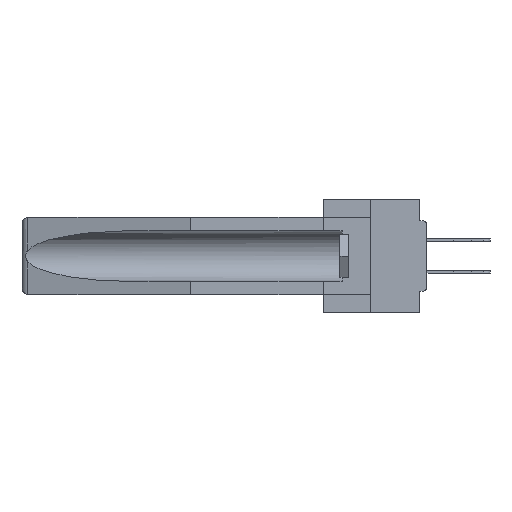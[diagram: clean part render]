
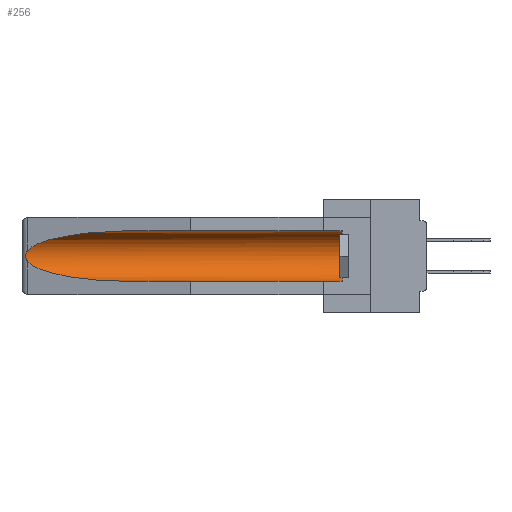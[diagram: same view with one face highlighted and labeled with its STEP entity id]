
A CAD part, left-side view. The second image highlights one B-rep face of the part: STEP entity #256.
In plain terms, the highlighted cylindrical face has radius 2.857 mm (diameter 5.715 mm), a partial arc.
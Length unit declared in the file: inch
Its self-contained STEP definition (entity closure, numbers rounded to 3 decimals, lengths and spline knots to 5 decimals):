
#256 = ADVANCED_FACE ( 'NONE', ( #24454 ), #22703, .F. ) ;
#654 = VERTEX_POINT ( 'NONE', #26336 ) ;
#983 = EDGE_CURVE ( 'NONE', #9670, #654, #21777, .T. ) ;
#1067 = LINE ( 'NONE', #14874, #6768 ) ;
#1359 = CARTESIAN_POINT ( 'NONE',  ( 0.26537, 1.52718, -0.14972 ) ) ;
#2585 = VERTEX_POINT ( 'NONE', #13475 ) ;
#2924 = CARTESIAN_POINT ( 'NONE',  ( 0.155, 0.126, -0.1715 ) ) ;
#4536 = CARTESIAN_POINT ( 'NONE',  ( 0.2675, 1.53308, -0.16763 ) ) ;
#6568 =( BOUNDED_CURVE ( )  B_SPLINE_CURVE ( 3, ( #15482, #18319, #7255, #1359 ),
 .UNSPECIFIED., .F., .F. ) 
 B_SPLINE_CURVE_WITH_KNOTS ( ( 4, 4 ),
 ( 4.71239, 6.08839 ),
 .UNSPECIFIED. ) 
 CURVE ( )  GEOMETRIC_REPRESENTATION_ITEM ( )  RATIONAL_B_SPLINE_CURVE ( ( 1., 0.848, 0.848, 1. ) ) 
 REPRESENTATION_ITEM ( '' )  );
#6768 = VECTOR ( 'NONE', #34058, 39.37008 ) ;
#7037 = DIRECTION ( 'NONE',  ( 0., 1., 0. ) ) ;
#7255 = CARTESIAN_POINT ( 'NONE',  ( 0.25451, 1.48313, -0.09465 ) ) ;
#8725 = CARTESIAN_POINT ( 'NONE',  ( 0.155, 0.126, -0.284 ) ) ;
#9670 = VERTEX_POINT ( 'NONE', #8725 ) ;
#9935 = CARTESIAN_POINT ( 'NONE',  ( 0.2675, 1.53308, -0.17534 ) ) ;
#10050 = CARTESIAN_POINT ( 'NONE',  ( 0.2673, 1.53269, -0.17917 ) ) ;
#10178 = CARTESIAN_POINT ( 'NONE',  ( 0.26654, 1.53092, -0.15636 ) ) ;
#10819 = EDGE_CURVE ( 'NONE', #2585, #19318, #11985, .T. ) ;
#11294 = DIRECTION ( 'NONE',  ( 0., -1., 0. ) ) ;
#11563 = ORIENTED_EDGE ( 'NONE', *, *, #10819, .T. ) ;
#11985 =( BOUNDED_CURVE ( )  B_SPLINE_CURVE ( 3, ( #14774, #20564, #17224, #28780 ),
 .UNSPECIFIED., .F., .F. ) 
 B_SPLINE_CURVE_WITH_KNOTS ( ( 4, 4 ),
 ( 0.1948, 1.5708 ),
 .UNSPECIFIED. ) 
 CURVE ( )  GEOMETRIC_REPRESENTATION_ITEM ( )  RATIONAL_B_SPLINE_CURVE ( ( 1., 0.848, 0.848, 1. ) ) 
 REPRESENTATION_ITEM ( '' )  );
#12118 = VERTEX_POINT ( 'NONE', #25406 ) ;
#12431 = AXIS2_PLACEMENT_3D ( 'NONE', #2924, #11294, #33782 ) ;
#12570 = CARTESIAN_POINT ( 'NONE',  ( 0.155, -0.30754, -0.059 ) ) ;
#13475 = CARTESIAN_POINT ( 'NONE',  ( 0.26537, 1.52718, -0.19328 ) ) ;
#14332 = AXIS2_PLACEMENT_3D ( 'NONE', #29173, #26584, #31389 ) ;
#14689 = ORIENTED_EDGE ( 'NONE', *, *, #23498, .T. ) ;
#14774 = CARTESIAN_POINT ( 'NONE',  ( 0.26537, 1.52718, -0.19328 ) ) ;
#14874 = CARTESIAN_POINT ( 'NONE',  ( 0.155, -0.30754, -0.284 ) ) ;
#15314 = ORIENTED_EDGE ( 'NONE', *, *, #983, .T. ) ;
#15482 = CARTESIAN_POINT ( 'NONE',  ( 0.155, 1.07973, -0.059 ) ) ;
#15732 = CARTESIAN_POINT ( 'NONE',  ( 0.26655, 1.53094, -0.18657 ) ) ;
#17224 = CARTESIAN_POINT ( 'NONE',  ( 0.21114, 1.30732, -0.284 ) ) ;
#17839 = ORIENTED_EDGE ( 'NONE', *, *, #25313, .F. ) ;
#18319 = CARTESIAN_POINT ( 'NONE',  ( 0.21114, 1.30732, -0.059 ) ) ;
#19318 = VERTEX_POINT ( 'NONE', #27812 ) ;
#20289 = EDGE_CURVE ( 'NONE', #12118, #2585, #26210, .T. ) ;
#20564 = CARTESIAN_POINT ( 'NONE',  ( 0.25451, 1.48313, -0.24835 ) ) ;
#21361 = EDGE_LOOP ( 'NONE', ( #14689, #34604, #11563, #17839, #15314, #36232 ) ) ;
#21521 = CARTESIAN_POINT ( 'NONE',  ( 0.26537, 1.52718, -0.14972 ) ) ;
#21640 = CARTESIAN_POINT ( 'NONE',  ( 0.155, 1.07973, -0.059 ) ) ;
#21777 = CIRCLE ( 'NONE', #12431, 0.1125 ) ;
#22703 = CYLINDRICAL_SURFACE ( 'NONE', #14332, 0.1125 ) ;
#23498 = EDGE_CURVE ( 'NONE', #23701, #12118, #6568, .T. ) ;
#23701 = VERTEX_POINT ( 'NONE', #21640 ) ;
#24454 = FACE_OUTER_BOUND ( 'NONE', #21361, .T. ) ;
#25313 = EDGE_CURVE ( 'NONE', #9670, #19318, #1067, .T. ) ;
#25406 = CARTESIAN_POINT ( 'NONE',  ( 0.26537, 1.52718, -0.14972 ) ) ;
#26210 = B_SPLINE_CURVE_WITH_KNOTS ( 'NONE', 3,
 ( #21521, #32697, #10178, #26901, #4536, #9935, #10050, #15732, #32572, #35422 ),
 .UNSPECIFIED., .F., .F.,
 ( 4, 2, 2, 2, 4 ),
 ( 0., 0.00029, 0.00058, 0.00087, 0.00117 ),
 .UNSPECIFIED. ) ;
#26336 = CARTESIAN_POINT ( 'NONE',  ( 0.155, 0.126, -0.059 ) ) ;
#26545 = VECTOR ( 'NONE', #7037, 39.37008 ) ;
#26584 = DIRECTION ( 'NONE',  ( 0., 1., 0. ) ) ;
#26901 = CARTESIAN_POINT ( 'NONE',  ( 0.2673, 1.5327, -0.16383 ) ) ;
#27414 = LINE ( 'NONE', #12570, #26545 ) ;
#27812 = CARTESIAN_POINT ( 'NONE',  ( 0.155, 1.07973, -0.284 ) ) ;
#28780 = CARTESIAN_POINT ( 'NONE',  ( 0.155, 1.07973, -0.284 ) ) ;
#29173 = CARTESIAN_POINT ( 'NONE',  ( 0.155, -0.30754, -0.1715 ) ) ;
#31389 = DIRECTION ( 'NONE',  ( 0., 0., 1. ) ) ;
#32572 = CARTESIAN_POINT ( 'NONE',  ( 0.26597, 1.5296, -0.19026 ) ) ;
#32697 = CARTESIAN_POINT ( 'NONE',  ( 0.26597, 1.52961, -0.15275 ) ) ;
#33782 = DIRECTION ( 'NONE',  ( 0., 0., 1. ) ) ;
#34058 = DIRECTION ( 'NONE',  ( 0., 1., 0. ) ) ;
#34343 = EDGE_CURVE ( 'NONE', #654, #23701, #27414, .T. ) ;
#34604 = ORIENTED_EDGE ( 'NONE', *, *, #20289, .T. ) ;
#35422 = CARTESIAN_POINT ( 'NONE',  ( 0.26537, 1.52718, -0.19328 ) ) ;
#36232 = ORIENTED_EDGE ( 'NONE', *, *, #34343, .T. ) ;
